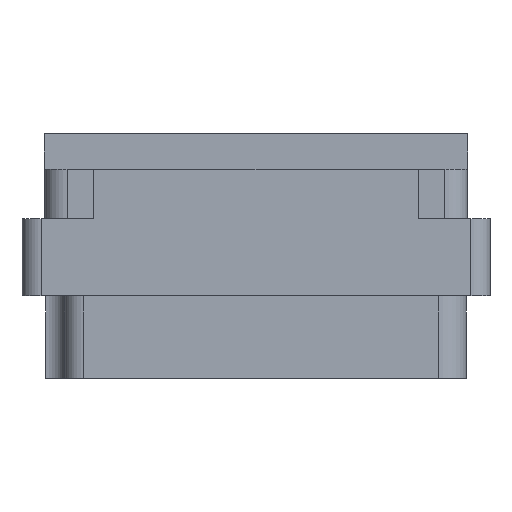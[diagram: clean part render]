
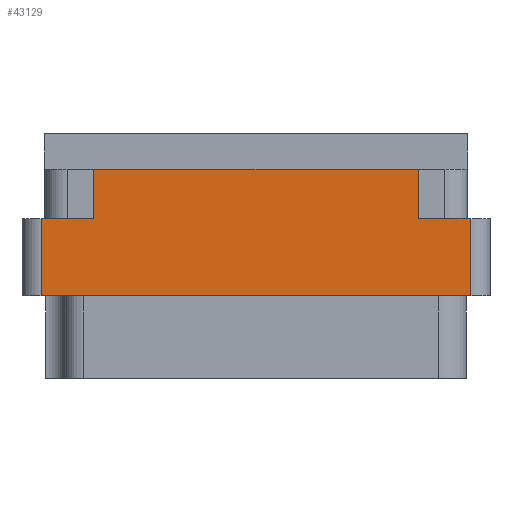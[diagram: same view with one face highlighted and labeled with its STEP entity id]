
A CAD part, left-side view. The second image highlights one B-rep face of the part: STEP entity #43129.
In plain terms, the highlighted planar face has unit normal (-1, 0, 0).
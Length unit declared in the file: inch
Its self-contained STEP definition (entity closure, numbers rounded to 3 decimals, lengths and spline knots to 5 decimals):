
#801 = FACE_OUTER_BOUND ( 'NONE', #48184, .T. ) ;
#2067 = EDGE_CURVE ( 'NONE', #66424, #25982, #40944, .T. ) ;
#4512 = VERTEX_POINT ( 'NONE', #19037 ) ;
#6897 = ORIENTED_EDGE ( 'NONE', *, *, #75968, .F. ) ;
#11490 = DIRECTION ( 'NONE',  ( 0., 1., 0. ) ) ;
#12884 = CARTESIAN_POINT ( 'NONE',  ( -1.375, 0.7005, -0.529 ) ) ;
#13884 = DIRECTION ( 'NONE',  ( 0., 0., -1. ) ) ;
#15691 = VECTOR ( 'NONE', #46035, 39.37008 ) ;
#15780 = EDGE_CURVE ( 'NONE', #46834, #4512, #45530, .T. ) ;
#17321 = CARTESIAN_POINT ( 'NONE',  ( -1.375, -0.5285, -0.277 ) ) ;
#18227 = EDGE_CURVE ( 'NONE', #79802, #66114, #33538, .T. ) ;
#18574 = CARTESIAN_POINT ( 'NONE',  ( -1.375, 0.5285, -0.277 ) ) ;
#18755 = CARTESIAN_POINT ( 'NONE',  ( -1.375, 0., -0.277 ) ) ;
#19037 = CARTESIAN_POINT ( 'NONE',  ( -1.375, 0.5285, -0.117 ) ) ;
#20200 = ORIENTED_EDGE ( 'NONE', *, *, #30232, .F. ) ;
#21937 = CARTESIAN_POINT ( 'NONE',  ( -1.375, -0.5285, -0.117 ) ) ;
#25048 = DIRECTION ( 'NONE',  ( 0., 0., 1. ) ) ;
#25982 = VERTEX_POINT ( 'NONE', #33114 ) ;
#28771 = CARTESIAN_POINT ( 'NONE',  ( -1.375, -0.5285, -0.277 ) ) ;
#29788 = ORIENTED_EDGE ( 'NONE', *, *, #57743, .T. ) ;
#30232 = EDGE_CURVE ( 'NONE', #4512, #66114, #49946, .T. ) ;
#31526 = PLANE ( 'NONE',  #80035 ) ;
#32886 = CARTESIAN_POINT ( 'NONE',  ( -1.375, 0., -0.277 ) ) ;
#33114 = CARTESIAN_POINT ( 'NONE',  ( -1.375, -0.7005, -0.277 ) ) ;
#33538 = LINE ( 'NONE', #17321, #76995 ) ;
#35489 = VECTOR ( 'NONE', #51552, 39.37008 ) ;
#40944 = LINE ( 'NONE', #59371, #15691 ) ;
#42418 = ORIENTED_EDGE ( 'NONE', *, *, #2067, .T. ) ;
#42580 = ORIENTED_EDGE ( 'NONE', *, *, #65900, .F. ) ;
#43129 = ADVANCED_FACE ( 'NONE', ( #801 ), #31526, .T. ) ;
#43800 = VECTOR ( 'NONE', #13884, 39.37008 ) ;
#43892 = LINE ( 'NONE', #86033, #43800 ) ;
#43953 = ORIENTED_EDGE ( 'NONE', *, *, #15780, .F. ) ;
#45530 = LINE ( 'NONE', #18574, #85807 ) ;
#46035 = DIRECTION ( 'NONE',  ( 0., 0., 1. ) ) ;
#46563 = VERTEX_POINT ( 'NONE', #12884 ) ;
#46798 = DIRECTION ( 'NONE',  ( 0., -1., 0. ) ) ;
#46834 = VERTEX_POINT ( 'NONE', #48806 ) ;
#48184 = EDGE_LOOP ( 'NONE', ( #6897, #29788, #83550, #42418, #42580, #87286, #20200, #43953 ) ) ;
#48806 = CARTESIAN_POINT ( 'NONE',  ( -1.375, 0.5285, -0.277 ) ) ;
#49946 = LINE ( 'NONE', #79128, #59462 ) ;
#51552 = DIRECTION ( 'NONE',  ( 0., -1., 0. ) ) ;
#51663 = CARTESIAN_POINT ( 'NONE',  ( -1.375, 0.7005, -0.277 ) ) ;
#55736 = EDGE_CURVE ( 'NONE', #66424, #46563, #79063, .T. ) ;
#56851 = VECTOR ( 'NONE', #46798, 39.37008 ) ;
#57743 = EDGE_CURVE ( 'NONE', #68430, #46563, #43892, .T. ) ;
#59294 = DIRECTION ( 'NONE',  ( 0., -1., 0. ) ) ;
#59371 = CARTESIAN_POINT ( 'NONE',  ( -1.375, -0.7005, -0.798 ) ) ;
#59462 = VECTOR ( 'NONE', #59294, 39.37008 ) ;
#61040 = VECTOR ( 'NONE', #11490, 39.37008 ) ;
#65316 = CARTESIAN_POINT ( 'NONE',  ( -1.375, -0.7625, -0.798 ) ) ;
#65900 = EDGE_CURVE ( 'NONE', #79802, #25982, #68461, .T. ) ;
#66114 = VERTEX_POINT ( 'NONE', #21937 ) ;
#66424 = VERTEX_POINT ( 'NONE', #71635 ) ;
#68430 = VERTEX_POINT ( 'NONE', #51663 ) ;
#68461 = LINE ( 'NONE', #32886, #56851 ) ;
#70234 = DIRECTION ( 'NONE',  ( 0., 0., 1. ) ) ;
#70533 = LINE ( 'NONE', #18755, #35489 ) ;
#71635 = CARTESIAN_POINT ( 'NONE',  ( -1.375, -0.7005, -0.529 ) ) ;
#75968 = EDGE_CURVE ( 'NONE', #68430, #46834, #70533, .T. ) ;
#76995 = VECTOR ( 'NONE', #70234, 39.37008 ) ;
#78912 = DIRECTION ( 'NONE',  ( -1., 0., 0. ) ) ;
#79063 = LINE ( 'NONE', #79426, #61040 ) ;
#79128 = CARTESIAN_POINT ( 'NONE',  ( -1.375, 0.7625, -0.117 ) ) ;
#79426 = CARTESIAN_POINT ( 'NONE',  ( -1.375, 0., -0.529 ) ) ;
#79802 = VERTEX_POINT ( 'NONE', #28771 ) ;
#80035 = AXIS2_PLACEMENT_3D ( 'NONE', #65316, #78912, #84251 ) ;
#83550 = ORIENTED_EDGE ( 'NONE', *, *, #55736, .F. ) ;
#84251 = DIRECTION ( 'NONE',  ( 0., 0., 1. ) ) ;
#85807 = VECTOR ( 'NONE', #25048, 39.37008 ) ;
#86033 = CARTESIAN_POINT ( 'NONE',  ( -1.375, 0.7005, -0.798 ) ) ;
#87286 = ORIENTED_EDGE ( 'NONE', *, *, #18227, .T. ) ;
